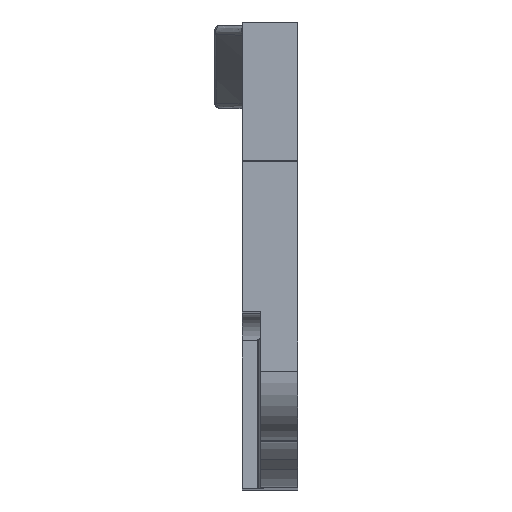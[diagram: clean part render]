
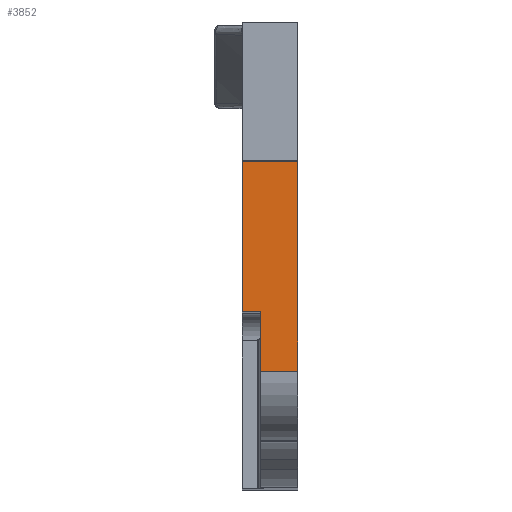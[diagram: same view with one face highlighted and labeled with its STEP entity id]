
A CAD part, top view. The second image highlights one B-rep face of the part: STEP entity #3852.
In plain terms, the highlighted planar face has unit normal (0, 0, 1).
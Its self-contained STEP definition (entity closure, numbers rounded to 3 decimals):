
#137 = EDGE_LOOP ( 'NONE', ( #2107, #2293, #1314, #522, #718, #1070 ) ) ;
#169 = DIRECTION ( 'NONE',  ( 0., -1., 0. ) ) ;
#224 = VERTEX_POINT ( 'NONE', #1966 ) ;
#231 = LINE ( 'NONE', #876, #2014 ) ;
#270 = VECTOR ( 'NONE', #1398, 1000. ) ;
#435 = VERTEX_POINT ( 'NONE', #3936 ) ;
#508 = LINE ( 'NONE', #1443, #270 ) ;
#522 = ORIENTED_EDGE ( 'NONE', *, *, #774, .F. ) ;
#718 = ORIENTED_EDGE ( 'NONE', *, *, #2121, .F. ) ;
#774 = EDGE_CURVE ( 'NONE', #435, #2736, #231, .T. ) ;
#876 = CARTESIAN_POINT ( 'NONE',  ( 0., 19.196, 3.82 ) ) ;
#931 = EDGE_CURVE ( 'NONE', #3217, #2736, #2492, .T. ) ;
#1028 = CARTESIAN_POINT ( 'NONE',  ( -2.675, 12.63, 3.82 ) ) ;
#1070 = ORIENTED_EDGE ( 'NONE', *, *, #3251, .F. ) ;
#1283 = DIRECTION ( 'NONE',  ( 0., 0., 1. ) ) ;
#1299 = VECTOR ( 'NONE', #1889, 1000. ) ;
#1314 = ORIENTED_EDGE ( 'NONE', *, *, #931, .T. ) ;
#1339 = CARTESIAN_POINT ( 'NONE',  ( 0., 8.346, 3.82 ) ) ;
#1367 = CARTESIAN_POINT ( 'NONE',  ( -4., 23.446, 3.82 ) ) ;
#1398 = DIRECTION ( 'NONE',  ( 0., 1., 0. ) ) ;
#1443 = CARTESIAN_POINT ( 'NONE',  ( -4., 19.196, 3.82 ) ) ;
#1452 = DIRECTION ( 'NONE',  ( 0., -1., 0. ) ) ;
#1795 = VERTEX_POINT ( 'NONE', #2733 ) ;
#1818 = CARTESIAN_POINT ( 'NONE',  ( -2.675, 8.346, 3.82 ) ) ;
#1889 = DIRECTION ( 'NONE',  ( 1., 0., 0. ) ) ;
#1966 = CARTESIAN_POINT ( 'NONE',  ( -2.675, 12.63, 3.82 ) ) ;
#2010 = EDGE_CURVE ( 'NONE', #3217, #224, #3028, .T. ) ;
#2014 = VECTOR ( 'NONE', #1452, 1000. ) ;
#2082 = EDGE_CURVE ( 'NONE', #224, #1795, #2804, .T. ) ;
#2096 = CARTESIAN_POINT ( 'NONE',  ( -2.675, 8.346, 3.82 ) ) ;
#2107 = ORIENTED_EDGE ( 'NONE', *, *, #2082, .F. ) ;
#2121 = EDGE_CURVE ( 'NONE', #3859, #435, #3774, .T. ) ;
#2259 = AXIS2_PLACEMENT_3D ( 'NONE', #3730, #1283, #169 ) ;
#2293 = ORIENTED_EDGE ( 'NONE', *, *, #2010, .F. ) ;
#2452 = CARTESIAN_POINT ( 'NONE',  ( -10., 8.346, 3.82 ) ) ;
#2492 = LINE ( 'NONE', #2452, #3509 ) ;
#2495 = PLANE ( 'NONE',  #2259 ) ;
#2733 = CARTESIAN_POINT ( 'NONE',  ( -4., 12.63, 3.82 ) ) ;
#2736 = VERTEX_POINT ( 'NONE', #1339 ) ;
#2804 = LINE ( 'NONE', #1028, #3180 ) ;
#2807 = FACE_OUTER_BOUND ( 'NONE', #137, .T. ) ;
#3028 = LINE ( 'NONE', #2096, #3438 ) ;
#3132 = CARTESIAN_POINT ( 'NONE',  ( -10., 23.446, 3.82 ) ) ;
#3168 = DIRECTION ( 'NONE',  ( -1., 0., 0. ) ) ;
#3180 = VECTOR ( 'NONE', #3168, 1000. ) ;
#3217 = VERTEX_POINT ( 'NONE', #1818 ) ;
#3251 = EDGE_CURVE ( 'NONE', #1795, #3859, #508, .T. ) ;
#3429 = DIRECTION ( 'NONE',  ( 1., 0., 0. ) ) ;
#3438 = VECTOR ( 'NONE', #3954, 1000. ) ;
#3509 = VECTOR ( 'NONE', #3429, 1000. ) ;
#3730 = CARTESIAN_POINT ( 'NONE',  ( -23.284, 19.196, 3.82 ) ) ;
#3774 = LINE ( 'NONE', #3132, #1299 ) ;
#3852 = ADVANCED_FACE ( 'NONE', ( #2807 ), #2495, .T. ) ;
#3859 = VERTEX_POINT ( 'NONE', #1367 ) ;
#3936 = CARTESIAN_POINT ( 'NONE',  ( 0., 23.446, 3.82 ) ) ;
#3954 = DIRECTION ( 'NONE',  ( 0., 1., 0. ) ) ;
